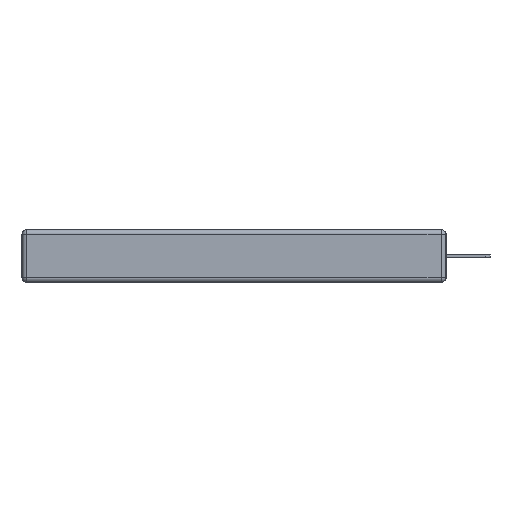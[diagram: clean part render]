
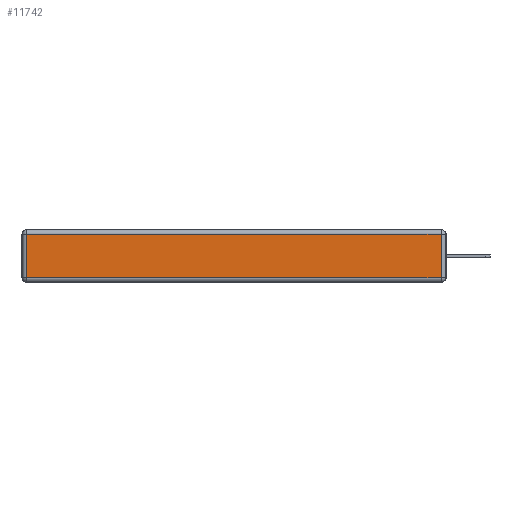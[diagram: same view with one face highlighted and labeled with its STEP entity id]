
A CAD part, left-side view. The second image highlights one B-rep face of the part: STEP entity #11742.
In plain terms, the highlighted planar face has unit normal (-1, 0, 0).
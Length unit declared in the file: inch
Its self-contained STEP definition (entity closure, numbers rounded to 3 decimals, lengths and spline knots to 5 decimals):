
#1678 = ORIENTED_EDGE ( 'NONE', *, *, #28022, .T. ) ;
#2373 = ORIENTED_EDGE ( 'NONE', *, *, #11519, .T. ) ;
#2803 = VERTEX_POINT ( 'NONE', #19338 ) ;
#3683 = VERTEX_POINT ( 'NONE', #12747 ) ;
#5740 = VECTOR ( 'NONE', #25258, 39.37008 ) ;
#7870 = LINE ( 'NONE', #21111, #18125 ) ;
#9087 = DIRECTION ( 'NONE',  ( 0., 0., -1. ) ) ;
#9526 = LINE ( 'NONE', #23082, #5740 ) ;
#9670 = DIRECTION ( 'NONE',  ( 0., 0., 1. ) ) ;
#10081 = DIRECTION ( 'NONE',  ( 0., -1., 0. ) ) ;
#10364 = ORIENTED_EDGE ( 'NONE', *, *, #27759, .T. ) ;
#11227 = LINE ( 'NONE', #13261, #17719 ) ;
#11410 = VERTEX_POINT ( 'NONE', #17026 ) ;
#11519 = EDGE_CURVE ( 'NONE', #11410, #3683, #17985, .T. ) ;
#11742 = ADVANCED_FACE ( 'NONE', ( #12485 ), #20603, .T. ) ;
#12164 = VECTOR ( 'NONE', #17490, 39.37008 ) ;
#12485 = FACE_OUTER_BOUND ( 'NONE', #25209, .T. ) ;
#12747 = CARTESIAN_POINT ( 'NONE',  ( 0., 2.72, -0.03 ) ) ;
#13261 = CARTESIAN_POINT ( 'NONE',  ( 0., 2.72, -0.343 ) ) ;
#14867 = EDGE_CURVE ( 'NONE', #28012, #2803, #7870, .T. ) ;
#15113 = ORIENTED_EDGE ( 'NONE', *, *, #14867, .T. ) ;
#16142 = CARTESIAN_POINT ( 'NONE',  ( 0., 0., -0.343 ) ) ;
#16434 = CARTESIAN_POINT ( 'NONE',  ( 0., 2.72, -0.313 ) ) ;
#17026 = CARTESIAN_POINT ( 'NONE',  ( 0., 0.03, -0.03 ) ) ;
#17490 = DIRECTION ( 'NONE',  ( 0., 1., 0. ) ) ;
#17719 = VECTOR ( 'NONE', #9087, 39.37008 ) ;
#17985 = LINE ( 'NONE', #23958, #12164 ) ;
#18125 = VECTOR ( 'NONE', #10081, 39.37008 ) ;
#19338 = CARTESIAN_POINT ( 'NONE',  ( 0., 0.03, -0.313 ) ) ;
#20603 = PLANE ( 'NONE',  #23772 ) ;
#21111 = CARTESIAN_POINT ( 'NONE',  ( 0., 0., -0.313 ) ) ;
#22809 = DIRECTION ( 'NONE',  ( -1., 0., 0. ) ) ;
#23082 = CARTESIAN_POINT ( 'NONE',  ( 0., 0.03, -0.343 ) ) ;
#23772 = AXIS2_PLACEMENT_3D ( 'NONE', #16142, #22809, #9670 ) ;
#23958 = CARTESIAN_POINT ( 'NONE',  ( 0., 2.75, -0.03 ) ) ;
#25209 = EDGE_LOOP ( 'NONE', ( #15113, #1678, #2373, #10364 ) ) ;
#25258 = DIRECTION ( 'NONE',  ( 0., 0., 1. ) ) ;
#27759 = EDGE_CURVE ( 'NONE', #3683, #28012, #11227, .T. ) ;
#28012 = VERTEX_POINT ( 'NONE', #16434 ) ;
#28022 = EDGE_CURVE ( 'NONE', #2803, #11410, #9526, .T. ) ;
